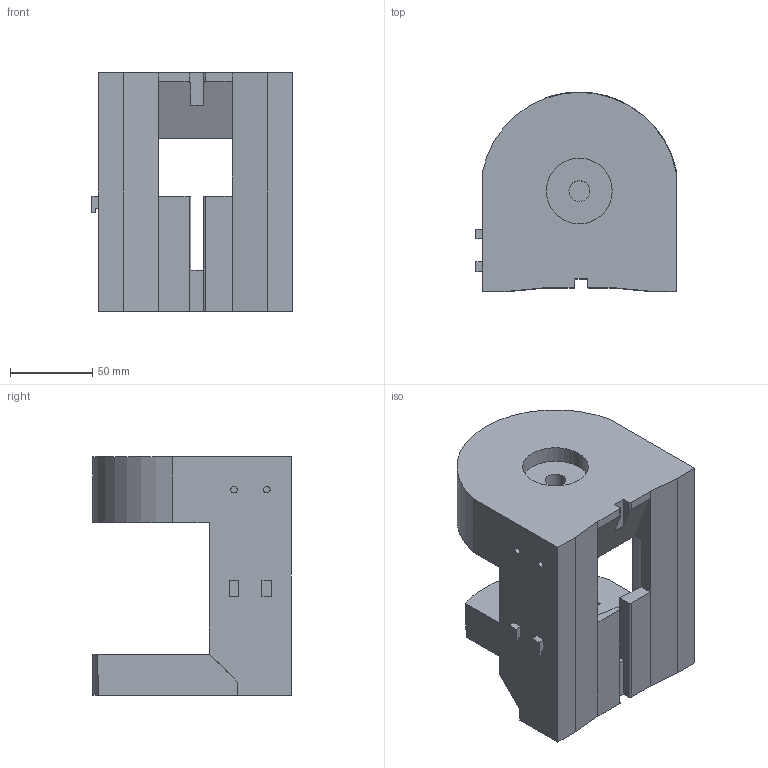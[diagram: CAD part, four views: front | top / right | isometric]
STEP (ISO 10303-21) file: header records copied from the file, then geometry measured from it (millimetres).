
FILE_DESCRIPTION (( 'STEP AP214' ), '1' );
FILE_NAME ('Normal Reciver Exstention.STEP', '2025-05-18T13:02:24', ( '' ), ( '' ), 'SwSTEP 2.0', 'SolidWorks 2024', '' );
FILE_SCHEMA (( 'AUTOMOTIVE_DESIGN' ));
Length unit declared in the file: millimetre
Products named in the file (1): Normal Reciver Exstention
Bounding box: 121.82 x 121 x 145 mm (x, y, z)
Volume: 877854.9 mm3; surface area: 105178.5 mm2
Topology: 1 solids, 1 shells, 99 faces, 273 edges, 180 vertices
Faces by surface type: plane 65, cylinder 32, cone 2
Entity records: 3260 total; most frequent: CARTESIAN_POINT 616, ORIENTED_EDGE 546, DIRECTION 546, EDGE_CURVE 273, LINE 186, VECTOR 186, AXIS2_PLACEMENT_3D 180, VERTEX_POINT 180
